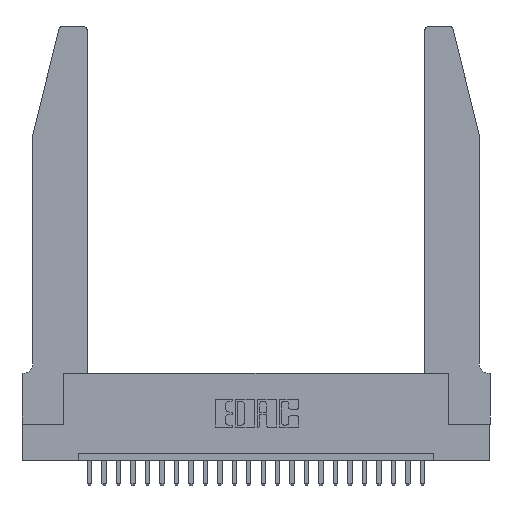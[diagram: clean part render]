
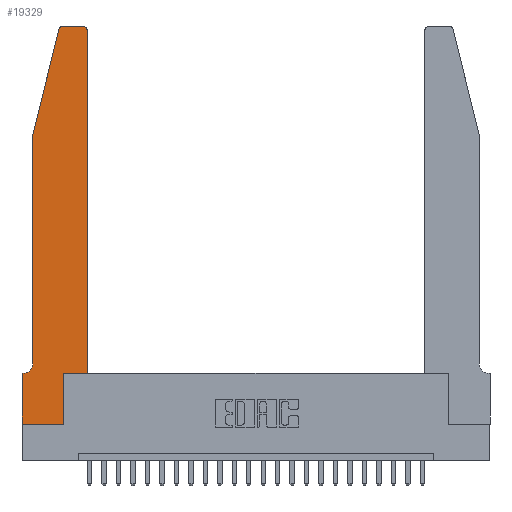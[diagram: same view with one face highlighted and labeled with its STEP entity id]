
A CAD part, top view. The second image highlights one B-rep face of the part: STEP entity #19329.
In plain terms, the highlighted planar face has unit normal (0, 0, 1).
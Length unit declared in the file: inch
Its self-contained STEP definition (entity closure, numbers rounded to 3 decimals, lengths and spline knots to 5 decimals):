
#54 = ORIENTED_EDGE ( 'NONE', *, *, #6262, .T. ) ;
#94 = ORIENTED_EDGE ( 'NONE', *, *, #20883, .T. ) ;
#244 = ORIENTED_EDGE ( 'NONE', *, *, #21852, .T. ) ;
#412 = CARTESIAN_POINT ( 'NONE',  ( 0.4505, 2.72, 0.37 ) ) ;
#576 = LINE ( 'NONE', #7010, #3942 ) ;
#667 = ORIENTED_EDGE ( 'NONE', *, *, #23575, .T. ) ;
#908 = EDGE_CURVE ( 'NONE', #7403, #18784, #21918, .T. ) ;
#1335 = DIRECTION ( 'NONE',  ( 0., 1., 0. ) ) ;
#1429 = VERTEX_POINT ( 'NONE', #3923 ) ;
#1578 = VERTEX_POINT ( 'NONE', #21320 ) ;
#1988 = DIRECTION ( 'NONE',  ( 0., 1., 0. ) ) ;
#1996 = DIRECTION ( 'NONE',  ( 0., 0., -1. ) ) ;
#2183 = VECTOR ( 'NONE', #18208, 39.37008 ) ;
#2274 = AXIS2_PLACEMENT_3D ( 'NONE', #14670, #10737, #8752 ) ;
#2380 = AXIS2_PLACEMENT_3D ( 'NONE', #10049, #1996, #23612 ) ;
#2395 = DIRECTION ( 'NONE',  ( 0., 0., 1. ) ) ;
#2547 = VECTOR ( 'NONE', #1988, 39.37008 ) ;
#2626 = EDGE_CURVE ( 'NONE', #14019, #7403, #4274, .T. ) ;
#2719 = ORIENTED_EDGE ( 'NONE', *, *, #6538, .T. ) ;
#3309 = LINE ( 'NONE', #9919, #9145 ) ;
#3715 = EDGE_CURVE ( 'NONE', #3796, #19831, #19660, .T. ) ;
#3796 = VERTEX_POINT ( 'NONE', #15350 ) ;
#3923 = CARTESIAN_POINT ( 'NONE',  ( 0., 0.35, 0.37 ) ) ;
#3942 = VECTOR ( 'NONE', #12844, 39.37008 ) ;
#3961 = VECTOR ( 'NONE', #21490, 39.37008 ) ;
#3984 = CIRCLE ( 'NONE', #2380, 0.07 ) ;
#4274 = LINE ( 'NONE', #5753, #18754 ) ;
#4493 = ORIENTED_EDGE ( 'NONE', *, *, #7958, .T. ) ;
#4719 = ORIENTED_EDGE ( 'NONE', *, *, #12849, .T. ) ;
#4730 = FACE_OUTER_BOUND ( 'NONE', #22166, .T. ) ;
#5383 = CARTESIAN_POINT ( 'NONE',  ( 0.4205, 2.75, 0.37 ) ) ;
#5753 = CARTESIAN_POINT ( 'NONE',  ( 0., 0., 0.37 ) ) ;
#6109 = VERTEX_POINT ( 'NONE', #11237 ) ;
#6159 = ORIENTED_EDGE ( 'NONE', *, *, #908, .T. ) ;
#6262 = EDGE_CURVE ( 'NONE', #18784, #3796, #12351, .T. ) ;
#6395 = AXIS2_PLACEMENT_3D ( 'NONE', #6736, #16784, #14998 ) ;
#6538 = EDGE_CURVE ( 'NONE', #1578, #1429, #24608, .T. ) ;
#6599 = CARTESIAN_POINT ( 'NONE',  ( 0., 0.35, 0.37 ) ) ;
#6736 = CARTESIAN_POINT ( 'NONE',  ( 0.4205, 2.72, 0.37 ) ) ;
#6775 = LINE ( 'NONE', #18294, #2183 ) ;
#6883 = CARTESIAN_POINT ( 'NONE',  ( 0.4505, 0.35, 0.37 ) ) ;
#6987 = DIRECTION ( 'NONE',  ( -1., 0., 0. ) ) ;
#7010 = CARTESIAN_POINT ( 'NONE',  ( 0.0755, 2., 0.37 ) ) ;
#7395 = VERTEX_POINT ( 'NONE', #24356 ) ;
#7403 = VERTEX_POINT ( 'NONE', #18649 ) ;
#7501 = CARTESIAN_POINT ( 'NONE',  ( 0.25487, 2.72718, 0.37 ) ) ;
#7937 = DIRECTION ( 'NONE',  ( -1., 0., 0. ) ) ;
#7948 = DIRECTION ( 'NONE',  ( 1., 0., 0. ) ) ;
#7958 = EDGE_CURVE ( 'NONE', #23762, #1578, #3984, .T. ) ;
#8493 = PLANE ( 'NONE',  #22818 ) ;
#8752 = DIRECTION ( 'NONE',  ( 1., 0., 0. ) ) ;
#9081 = CARTESIAN_POINT ( 'NONE',  ( 0.0755, 0.42, 0.37 ) ) ;
#9145 = VECTOR ( 'NONE', #7937, 39.37008 ) ;
#9484 = CARTESIAN_POINT ( 'NONE',  ( 0., 0., 0.37 ) ) ;
#9919 = CARTESIAN_POINT ( 'NONE',  ( 0.2605, 2.75, 0.37 ) ) ;
#10049 = CARTESIAN_POINT ( 'NONE',  ( 0.0055, 0.42, 0.37 ) ) ;
#10201 = VECTOR ( 'NONE', #6987, 39.37008 ) ;
#10737 = DIRECTION ( 'NONE',  ( 0., 0., 1. ) ) ;
#11024 = VECTOR ( 'NONE', #1335, 39.37008 ) ;
#11237 = CARTESIAN_POINT ( 'NONE',  ( 0.0755, 2., 0.37 ) ) ;
#11525 = CARTESIAN_POINT ( 'NONE',  ( 0.0755, 2., 0.37 ) ) ;
#11762 = VECTOR ( 'NONE', #7948, 39.37008 ) ;
#12351 = LINE ( 'NONE', #19366, #11762 ) ;
#12844 = DIRECTION ( 'NONE',  ( -0.239, -0.971, 0. ) ) ;
#12849 = EDGE_CURVE ( 'NONE', #19831, #17402, #14529, .T. ) ;
#12927 = CIRCLE ( 'NONE', #2274, 0.03 ) ;
#14019 = VERTEX_POINT ( 'NONE', #9484 ) ;
#14529 = CIRCLE ( 'NONE', #6395, 0.03 ) ;
#14670 = CARTESIAN_POINT ( 'NONE',  ( 0.284, 2.72, 0.37 ) ) ;
#14998 = DIRECTION ( 'NONE',  ( 1., 0., 0. ) ) ;
#15252 = ORIENTED_EDGE ( 'NONE', *, *, #2626, .T. ) ;
#15350 = CARTESIAN_POINT ( 'NONE',  ( 0.4505, 0.35, 0.37 ) ) ;
#15841 = ORIENTED_EDGE ( 'NONE', *, *, #3715, .T. ) ;
#16677 = CARTESIAN_POINT ( 'NONE',  ( 0.0755, 0.35, 0.37 ) ) ;
#16784 = DIRECTION ( 'NONE',  ( 0., 0., 1. ) ) ;
#17402 = VERTEX_POINT ( 'NONE', #5383 ) ;
#17526 = ORIENTED_EDGE ( 'NONE', *, *, #23166, .T. ) ;
#17578 = DIRECTION ( 'NONE',  ( 1., 0., 0. ) ) ;
#18208 = DIRECTION ( 'NONE',  ( 0., -1., 0. ) ) ;
#18294 = CARTESIAN_POINT ( 'NONE',  ( 0., 0., 0.37 ) ) ;
#18649 = CARTESIAN_POINT ( 'NONE',  ( 0.2865, 0., 0.37 ) ) ;
#18754 = VECTOR ( 'NONE', #17578, 39.37008 ) ;
#18784 = VERTEX_POINT ( 'NONE', #22109 ) ;
#19329 = ADVANCED_FACE ( 'NONE', ( #4730 ), #8493, .T. ) ;
#19366 = CARTESIAN_POINT ( 'NONE',  ( 0.4505, 0.35, 0.37 ) ) ;
#19660 = LINE ( 'NONE', #6883, #11024 ) ;
#19831 = VERTEX_POINT ( 'NONE', #412 ) ;
#20763 = ORIENTED_EDGE ( 'NONE', *, *, #23912, .T. ) ;
#20883 = EDGE_CURVE ( 'NONE', #1429, #14019, #6775, .T. ) ;
#21320 = CARTESIAN_POINT ( 'NONE',  ( 0.0055, 0.35, 0.37 ) ) ;
#21490 = DIRECTION ( 'NONE',  ( 0., -1., 0. ) ) ;
#21575 = CARTESIAN_POINT ( 'NONE',  ( 0.2865, 0.35, 0.37 ) ) ;
#21852 = EDGE_CURVE ( 'NONE', #7395, #24300, #12927, .T. ) ;
#21918 = LINE ( 'NONE', #21575, #2547 ) ;
#22109 = CARTESIAN_POINT ( 'NONE',  ( 0.2865, 0.35, 0.37 ) ) ;
#22134 = DIRECTION ( 'NONE',  ( 1., 0., 0. ) ) ;
#22166 = EDGE_LOOP ( 'NONE', ( #20763, #244, #667, #17526, #4493, #2719, #94, #15252, #6159, #54, #15841, #4719 ) ) ;
#22706 = LINE ( 'NONE', #11525, #3961 ) ;
#22818 = AXIS2_PLACEMENT_3D ( 'NONE', #6599, #2395, #22134 ) ;
#23166 = EDGE_CURVE ( 'NONE', #6109, #23762, #22706, .T. ) ;
#23575 = EDGE_CURVE ( 'NONE', #24300, #6109, #576, .T. ) ;
#23612 = DIRECTION ( 'NONE',  ( -1., 0., 0. ) ) ;
#23762 = VERTEX_POINT ( 'NONE', #9081 ) ;
#23912 = EDGE_CURVE ( 'NONE', #17402, #7395, #3309, .T. ) ;
#24300 = VERTEX_POINT ( 'NONE', #7501 ) ;
#24356 = CARTESIAN_POINT ( 'NONE',  ( 0.284, 2.75, 0.37 ) ) ;
#24608 = LINE ( 'NONE', #16677, #10201 ) ;
